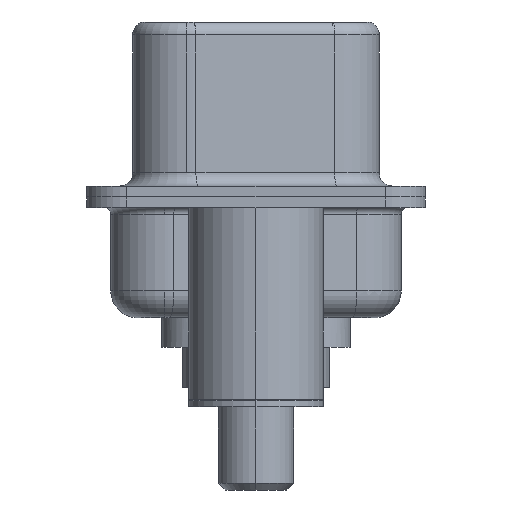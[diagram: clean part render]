
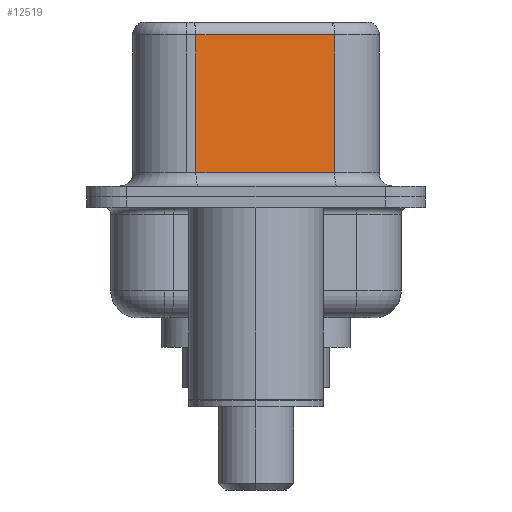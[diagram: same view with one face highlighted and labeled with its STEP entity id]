
A CAD part, left-side view. The second image highlights one B-rep face of the part: STEP entity #12519.
In plain terms, the highlighted planar face has unit normal (-0.985, -0.174, 0).
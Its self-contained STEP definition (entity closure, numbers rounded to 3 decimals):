
#214 = PLANE ( 'NONE',  #1382 ) ;
#1382 = AXIS2_PLACEMENT_3D ( 'NONE', #6670, #5478, #1647 ) ;
#1647 = DIRECTION ( 'NONE',  ( -0.174, 0.985, 0. ) ) ;
#1840 = CARTESIAN_POINT ( 'NONE',  ( 3.67, 2.233, 6.02 ) ) ;
#3195 = EDGE_LOOP ( 'NONE', ( #6320, #5079, #14156, #15277 ) ) ;
#3675 = DIRECTION ( 'NONE',  ( 0.174, -0.985, 0. ) ) ;
#3774 = VERTEX_POINT ( 'NONE', #12697 ) ;
#3795 = LINE ( 'NONE', #14758, #10240 ) ;
#4126 = EDGE_CURVE ( 'NONE', #8552, #7109, #13942, .T. ) ;
#4819 = VERTEX_POINT ( 'NONE', #1840 ) ;
#5079 = ORIENTED_EDGE ( 'NONE', *, *, #5226, .T. ) ;
#5226 = EDGE_CURVE ( 'NONE', #8552, #4819, #5395, .T. ) ;
#5395 = LINE ( 'NONE', #6229, #10103 ) ;
#5478 = DIRECTION ( 'NONE',  ( 0.985, 0.174, 0. ) ) ;
#6091 = CARTESIAN_POINT ( 'NONE',  ( 4.58, -2.927, 6.52 ) ) ;
#6229 = CARTESIAN_POINT ( 'NONE',  ( 4.58, -2.927, 6.02 ) ) ;
#6320 = ORIENTED_EDGE ( 'NONE', *, *, #4126, .F. ) ;
#6385 = CARTESIAN_POINT ( 'NONE',  ( 4.58, -2.927, 0.9 ) ) ;
#6670 = CARTESIAN_POINT ( 'NONE',  ( 4.58, -2.927, 6.52 ) ) ;
#6756 = EDGE_CURVE ( 'NONE', #4819, #3774, #3795, .T. ) ;
#7109 = VERTEX_POINT ( 'NONE', #11369 ) ;
#7469 = VECTOR ( 'NONE', #3675, 1000. ) ;
#8552 = VERTEX_POINT ( 'NONE', #13330 ) ;
#9513 = DIRECTION ( 'NONE',  ( 0., 0., -1. ) ) ;
#9816 = EDGE_CURVE ( 'NONE', #3774, #7109, #16132, .T. ) ;
#9824 = DIRECTION ( 'NONE',  ( 0., 0., -1. ) ) ;
#10103 = VECTOR ( 'NONE', #10881, 1000. ) ;
#10240 = VECTOR ( 'NONE', #9513, 1000. ) ;
#10881 = DIRECTION ( 'NONE',  ( -0.174, 0.985, 0. ) ) ;
#11369 = CARTESIAN_POINT ( 'NONE',  ( 4.58, -2.927, 0.9 ) ) ;
#12519 = ADVANCED_FACE ( 'NONE', ( #12969 ), #214, .F. ) ;
#12697 = CARTESIAN_POINT ( 'NONE',  ( 3.67, 2.233, 0.9 ) ) ;
#12969 = FACE_OUTER_BOUND ( 'NONE', #3195, .T. ) ;
#13330 = CARTESIAN_POINT ( 'NONE',  ( 4.58, -2.927, 6.02 ) ) ;
#13942 = LINE ( 'NONE', #6091, #14125 ) ;
#14125 = VECTOR ( 'NONE', #9824, 1000. ) ;
#14156 = ORIENTED_EDGE ( 'NONE', *, *, #6756, .T. ) ;
#14758 = CARTESIAN_POINT ( 'NONE',  ( 3.67, 2.233, 6.52 ) ) ;
#15277 = ORIENTED_EDGE ( 'NONE', *, *, #9816, .T. ) ;
#16132 = LINE ( 'NONE', #6385, #7469 ) ;
